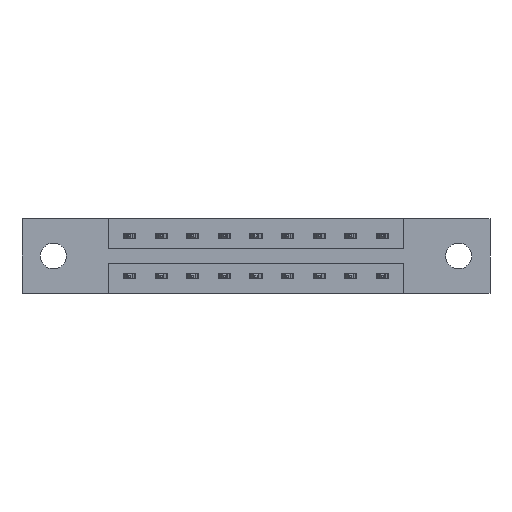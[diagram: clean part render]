
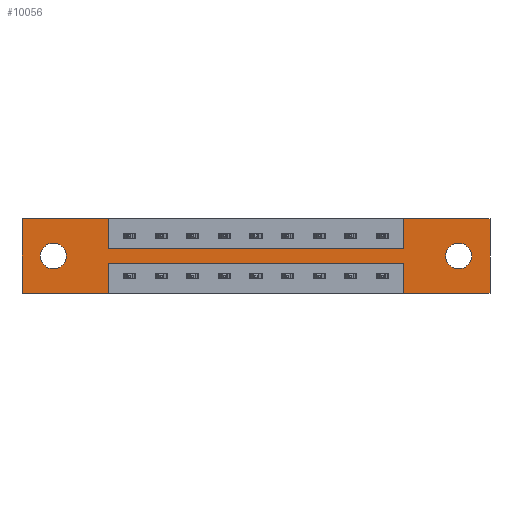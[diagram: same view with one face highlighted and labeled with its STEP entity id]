
A CAD part, front view. The second image highlights one B-rep face of the part: STEP entity #10056.
In plain terms, the highlighted planar face has unit normal (0, -1, 0).
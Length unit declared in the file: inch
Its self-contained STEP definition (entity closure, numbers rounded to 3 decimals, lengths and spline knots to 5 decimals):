
#73 = VECTOR ( 'NONE', #2866, 39.37008 ) ;
#122 = EDGE_CURVE ( 'NONE', #2382, #3497, #3740, .T. ) ;
#143 = ORIENTED_EDGE ( 'NONE', *, *, #2209, .T. ) ;
#276 = DIRECTION ( 'NONE',  ( 0., 0., 1. ) ) ;
#295 = VERTEX_POINT ( 'NONE', #4883 ) ;
#322 = DIRECTION ( 'NONE',  ( 0., 1., 0. ) ) ;
#379 = FACE_BOUND ( 'NONE', #10109, .T. ) ;
#387 = LINE ( 'NONE', #2836, #73 ) ;
#432 = AXIS2_PLACEMENT_3D ( 'NONE', #1966, #2695, #5552 ) ;
#582 = ORIENTED_EDGE ( 'NONE', *, *, #9228, .F. ) ;
#764 = LINE ( 'NONE', #2420, #5539 ) ;
#845 = EDGE_CURVE ( 'NONE', #5896, #8103, #3634, .T. ) ;
#954 = DIRECTION ( 'NONE',  ( 0., 0., 1. ) ) ;
#1220 = LINE ( 'NONE', #9103, #6234 ) ;
#1345 = VECTOR ( 'NONE', #7973, 39.37008 ) ;
#1354 = ORIENTED_EDGE ( 'NONE', *, *, #3678, .F. ) ;
#1448 = DIRECTION ( 'NONE',  ( -1., 0., 0. ) ) ;
#1729 = CARTESIAN_POINT ( 'NONE',  ( 0.425, 0., -0.15 ) ) ;
#1796 = CARTESIAN_POINT ( 'NONE',  ( 1.885, 0., -0.15 ) ) ;
#1804 = FACE_OUTER_BOUND ( 'NONE', #5736, .T. ) ;
#1965 = DIRECTION ( 'NONE',  ( 1., 0., 0. ) ) ;
#1966 = CARTESIAN_POINT ( 'NONE',  ( 2.155, 0., -0.185 ) ) ;
#2017 = CARTESIAN_POINT ( 'NONE',  ( 0., 0., 0. ) ) ;
#2080 = VERTEX_POINT ( 'NONE', #9365 ) ;
#2095 = CARTESIAN_POINT ( 'NONE',  ( 0., 0., 0. ) ) ;
#2197 = ORIENTED_EDGE ( 'NONE', *, *, #122, .F. ) ;
#2209 = EDGE_CURVE ( 'NONE', #2751, #3331, #6128, .T. ) ;
#2212 = ORIENTED_EDGE ( 'NONE', *, *, #845, .T. ) ;
#2382 = VERTEX_POINT ( 'NONE', #3099 ) ;
#2420 = CARTESIAN_POINT ( 'NONE',  ( 0.425, 0., -0.15 ) ) ;
#2602 = AXIS2_PLACEMENT_3D ( 'NONE', #9548, #3614, #9581 ) ;
#2669 = PLANE ( 'NONE',  #2602 ) ;
#2695 = DIRECTION ( 'NONE',  ( 0., 1., 0. ) ) ;
#2745 = LINE ( 'NONE', #9448, #4944 ) ;
#2751 = VERTEX_POINT ( 'NONE', #8546 ) ;
#2836 = CARTESIAN_POINT ( 'NONE',  ( 2.31, 0., 0. ) ) ;
#2866 = DIRECTION ( 'NONE',  ( 0., 0., -1. ) ) ;
#2928 = VERTEX_POINT ( 'NONE', #9096 ) ;
#2960 = VERTEX_POINT ( 'NONE', #1796 ) ;
#3099 = CARTESIAN_POINT ( 'NONE',  ( 0.425, 0., -0.37 ) ) ;
#3194 = CARTESIAN_POINT ( 'NONE',  ( 0., 0., -0.37 ) ) ;
#3213 = EDGE_LOOP ( 'NONE', ( #143, #7732 ) ) ;
#3331 = VERTEX_POINT ( 'NONE', #10495 ) ;
#3480 = EDGE_CURVE ( 'NONE', #10891, #10734, #9081, .T. ) ;
#3497 = VERTEX_POINT ( 'NONE', #10617 ) ;
#3504 = DIRECTION ( 'NONE',  ( 0., 0., -1. ) ) ;
#3568 = EDGE_CURVE ( 'NONE', #6020, #2960, #764, .T. ) ;
#3591 = DIRECTION ( 'NONE',  ( 0., 0., 1. ) ) ;
#3614 = DIRECTION ( 'NONE',  ( 0., -1., 0. ) ) ;
#3634 = CIRCLE ( 'NONE', #7123, 0.064 ) ;
#3678 = EDGE_CURVE ( 'NONE', #2928, #2382, #7279, .T. ) ;
#3740 = LINE ( 'NONE', #3194, #10195 ) ;
#3773 = CARTESIAN_POINT ( 'NONE',  ( 0., 0., -0.37 ) ) ;
#3830 = CARTESIAN_POINT ( 'NONE',  ( 0.155, 0., -0.185 ) ) ;
#4029 = EDGE_CURVE ( 'NONE', #3331, #2751, #10160, .T. ) ;
#4146 = VERTEX_POINT ( 'NONE', #2017 ) ;
#4200 = EDGE_CURVE ( 'NONE', #295, #6020, #1220, .T. ) ;
#4234 = DIRECTION ( 'NONE',  ( -1., 0., 0. ) ) ;
#4444 = DIRECTION ( 'NONE',  ( 0., 0., 1. ) ) ;
#4883 = CARTESIAN_POINT ( 'NONE',  ( 0.425, 0., 0. ) ) ;
#4944 = VECTOR ( 'NONE', #4444, 39.37008 ) ;
#5152 = ORIENTED_EDGE ( 'NONE', *, *, #4200, .F. ) ;
#5206 = EDGE_CURVE ( 'NONE', #2080, #8638, #10590, .T. ) ;
#5242 = ORIENTED_EDGE ( 'NONE', *, *, #5940, .F. ) ;
#5312 = EDGE_CURVE ( 'NONE', #8638, #10891, #387, .T. ) ;
#5348 = CARTESIAN_POINT ( 'NONE',  ( 0., 0., 0. ) ) ;
#5539 = VECTOR ( 'NONE', #9971, 39.37008 ) ;
#5552 = DIRECTION ( 'NONE',  ( 0., 0., -1. ) ) ;
#5613 = VERTEX_POINT ( 'NONE', #11067 ) ;
#5690 = CARTESIAN_POINT ( 'NONE',  ( 2.31, 0., -0.37 ) ) ;
#5736 = EDGE_LOOP ( 'NONE', ( #1354, #8639, #9253, #9869, #8377, #9035, #7210, #7422, #5152, #5242, #582, #2197 ) ) ;
#5782 = DIRECTION ( 'NONE',  ( 0., 0., 1. ) ) ;
#5896 = VERTEX_POINT ( 'NONE', #9765 ) ;
#5940 = EDGE_CURVE ( 'NONE', #4146, #295, #8282, .T. ) ;
#6020 = VERTEX_POINT ( 'NONE', #1729 ) ;
#6128 = CIRCLE ( 'NONE', #9184, 0.064 ) ;
#6234 = VECTOR ( 'NONE', #3504, 39.37008 ) ;
#6369 = CARTESIAN_POINT ( 'NONE',  ( 0.425, 0., -0.37 ) ) ;
#6412 = EDGE_CURVE ( 'NONE', #8103, #5896, #6604, .T. ) ;
#6430 = CARTESIAN_POINT ( 'NONE',  ( 1.885, 0., -0.37 ) ) ;
#6498 = LINE ( 'NONE', #8260, #10502 ) ;
#6523 = AXIS2_PLACEMENT_3D ( 'NONE', #3830, #322, #276 ) ;
#6604 = CIRCLE ( 'NONE', #432, 0.064 ) ;
#6730 = FACE_BOUND ( 'NONE', #3213, .T. ) ;
#6879 = EDGE_CURVE ( 'NONE', #5613, #2928, #7161, .T. ) ;
#6903 = VECTOR ( 'NONE', #7522, 39.37008 ) ;
#6905 = VECTOR ( 'NONE', #1448, 39.37008 ) ;
#6907 = CARTESIAN_POINT ( 'NONE',  ( 2.155, 0., -0.185 ) ) ;
#7026 = VECTOR ( 'NONE', #9984, 39.37008 ) ;
#7123 = AXIS2_PLACEMENT_3D ( 'NONE', #6907, #10380, #8621 ) ;
#7161 = LINE ( 'NONE', #10878, #6903 ) ;
#7210 = ORIENTED_EDGE ( 'NONE', *, *, #10517, .F. ) ;
#7279 = LINE ( 'NONE', #6369, #7026 ) ;
#7293 = ORIENTED_EDGE ( 'NONE', *, *, #6412, .T. ) ;
#7422 = ORIENTED_EDGE ( 'NONE', *, *, #3568, .F. ) ;
#7476 = VECTOR ( 'NONE', #3591, 39.37008 ) ;
#7522 = DIRECTION ( 'NONE',  ( -1., 0., 0. ) ) ;
#7591 = EDGE_CURVE ( 'NONE', #10734, #5613, #6498, .T. ) ;
#7732 = ORIENTED_EDGE ( 'NONE', *, *, #4029, .T. ) ;
#7973 = DIRECTION ( 'NONE',  ( 1., 0., 0. ) ) ;
#8103 = VERTEX_POINT ( 'NONE', #11269 ) ;
#8260 = CARTESIAN_POINT ( 'NONE',  ( 1.885, 0., -0.37 ) ) ;
#8282 = LINE ( 'NONE', #2095, #10136 ) ;
#8377 = ORIENTED_EDGE ( 'NONE', *, *, #5312, .F. ) ;
#8546 = CARTESIAN_POINT ( 'NONE',  ( 0.155, 0., -0.121 ) ) ;
#8621 = DIRECTION ( 'NONE',  ( 0., 0., -1. ) ) ;
#8638 = VERTEX_POINT ( 'NONE', #10460 ) ;
#8639 = ORIENTED_EDGE ( 'NONE', *, *, #6879, .F. ) ;
#8995 = CARTESIAN_POINT ( 'NONE',  ( 0.155, 0., -0.185 ) ) ;
#9035 = ORIENTED_EDGE ( 'NONE', *, *, #5206, .F. ) ;
#9081 = LINE ( 'NONE', #3773, #6905 ) ;
#9096 = CARTESIAN_POINT ( 'NONE',  ( 0.425, 0., -0.22 ) ) ;
#9103 = CARTESIAN_POINT ( 'NONE',  ( 0.425, 0., 0. ) ) ;
#9184 = AXIS2_PLACEMENT_3D ( 'NONE', #8995, #10353, #954 ) ;
#9228 = EDGE_CURVE ( 'NONE', #3497, #4146, #9634, .T. ) ;
#9253 = ORIENTED_EDGE ( 'NONE', *, *, #7591, .F. ) ;
#9365 = CARTESIAN_POINT ( 'NONE',  ( 1.885, 0., 0. ) ) ;
#9448 = CARTESIAN_POINT ( 'NONE',  ( 1.885, 0., 0. ) ) ;
#9548 = CARTESIAN_POINT ( 'NONE',  ( 0., 0., -0.37 ) ) ;
#9581 = DIRECTION ( 'NONE',  ( 0., 0., -1. ) ) ;
#9634 = LINE ( 'NONE', #5348, #7476 ) ;
#9765 = CARTESIAN_POINT ( 'NONE',  ( 2.155, 0., -0.121 ) ) ;
#9869 = ORIENTED_EDGE ( 'NONE', *, *, #3480, .F. ) ;
#9971 = DIRECTION ( 'NONE',  ( 1., 0., 0. ) ) ;
#9984 = DIRECTION ( 'NONE',  ( 0., 0., -1. ) ) ;
#10056 = ADVANCED_FACE ( 'NONE', ( #379, #6730, #1804 ), #2669, .T. ) ;
#10109 = EDGE_LOOP ( 'NONE', ( #2212, #7293 ) ) ;
#10136 = VECTOR ( 'NONE', #1965, 39.37008 ) ;
#10160 = CIRCLE ( 'NONE', #6523, 0.064 ) ;
#10195 = VECTOR ( 'NONE', #4234, 39.37008 ) ;
#10353 = DIRECTION ( 'NONE',  ( 0., 1., 0. ) ) ;
#10380 = DIRECTION ( 'NONE',  ( 0., 1., 0. ) ) ;
#10460 = CARTESIAN_POINT ( 'NONE',  ( 2.31, 0., 0. ) ) ;
#10471 = CARTESIAN_POINT ( 'NONE',  ( 0., 0., 0. ) ) ;
#10495 = CARTESIAN_POINT ( 'NONE',  ( 0.155, 0., -0.249 ) ) ;
#10502 = VECTOR ( 'NONE', #5782, 39.37008 ) ;
#10517 = EDGE_CURVE ( 'NONE', #2960, #2080, #2745, .T. ) ;
#10590 = LINE ( 'NONE', #10471, #1345 ) ;
#10617 = CARTESIAN_POINT ( 'NONE',  ( 0., 0., -0.37 ) ) ;
#10734 = VERTEX_POINT ( 'NONE', #6430 ) ;
#10878 = CARTESIAN_POINT ( 'NONE',  ( 0.425, 0., -0.22 ) ) ;
#10891 = VERTEX_POINT ( 'NONE', #5690 ) ;
#11067 = CARTESIAN_POINT ( 'NONE',  ( 1.885, 0., -0.22 ) ) ;
#11269 = CARTESIAN_POINT ( 'NONE',  ( 2.155, 0., -0.249 ) ) ;
